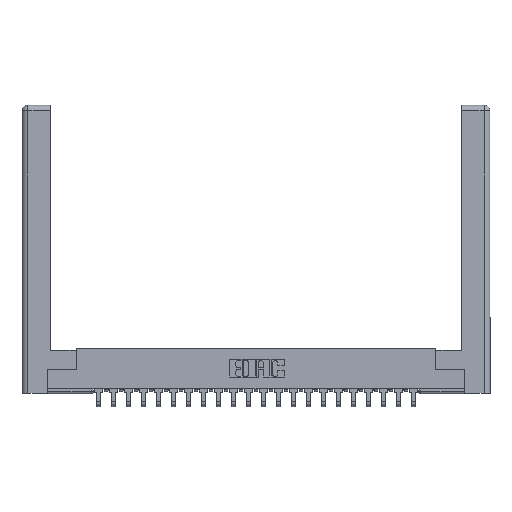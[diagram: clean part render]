
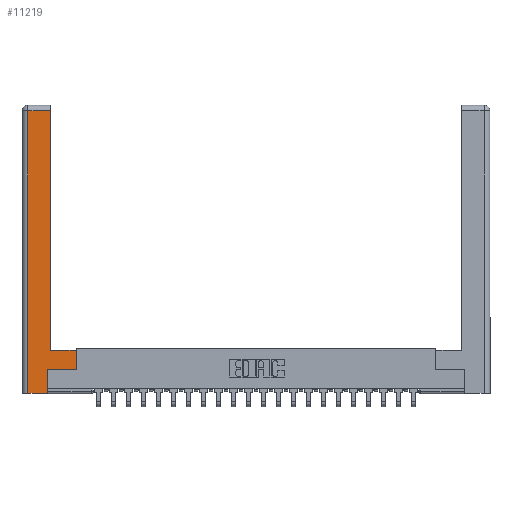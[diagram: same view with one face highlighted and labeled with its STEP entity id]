
A CAD part, top view. The second image highlights one B-rep face of the part: STEP entity #11219.
In plain terms, the highlighted planar face has unit normal (0, 0, 1).
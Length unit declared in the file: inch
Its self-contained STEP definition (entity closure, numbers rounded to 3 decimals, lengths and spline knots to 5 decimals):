
#249 = CARTESIAN_POINT ( 'NONE',  ( 0.265, 0.245, 0. ) ) ;
#416 = VECTOR ( 'NONE', #13026, 39.37008 ) ;
#850 = DIRECTION ( 'NONE',  ( 0., 1., 0. ) ) ;
#960 = VECTOR ( 'NONE', #8454, 39.37008 ) ;
#1880 = ORIENTED_EDGE ( 'NONE', *, *, #22420, .T. ) ;
#1926 = CARTESIAN_POINT ( 'NONE',  ( 0.295, 2.94, 0. ) ) ;
#2036 = LINE ( 'NONE', #17724, #17141 ) ;
#2659 = ORIENTED_EDGE ( 'NONE', *, *, #13560, .T. ) ;
#2972 = DIRECTION ( 'NONE',  ( 1., 0., 0. ) ) ;
#3571 = EDGE_CURVE ( 'NONE', #18539, #9554, #7698, .T. ) ;
#4336 = DIRECTION ( 'NONE',  ( 1., 0., 0. ) ) ;
#4462 = VERTEX_POINT ( 'NONE', #1926 ) ;
#5749 = ORIENTED_EDGE ( 'NONE', *, *, #9515, .T. ) ;
#5906 = LINE ( 'NONE', #19594, #960 ) ;
#6260 = EDGE_CURVE ( 'NONE', #16637, #12962, #2036, .T. ) ;
#6638 = CARTESIAN_POINT ( 'NONE',  ( 0.0615, 0., 0. ) ) ;
#6993 = LINE ( 'NONE', #19437, #16302 ) ;
#7064 = ORIENTED_EDGE ( 'NONE', *, *, #6260, .T. ) ;
#7620 = VECTOR ( 'NONE', #4336, 39.37008 ) ;
#7698 = LINE ( 'NONE', #11006, #416 ) ;
#7737 = CARTESIAN_POINT ( 'NONE',  ( 0.0615, 0., 0. ) ) ;
#8075 = LINE ( 'NONE', #16830, #17654 ) ;
#8365 = VERTEX_POINT ( 'NONE', #20976 ) ;
#8407 = ORIENTED_EDGE ( 'NONE', *, *, #18143, .T. ) ;
#8454 = DIRECTION ( 'NONE',  ( -1., 0., 0. ) ) ;
#9093 = VECTOR ( 'NONE', #23671, 39.37008 ) ;
#9161 = VERTEX_POINT ( 'NONE', #6638 ) ;
#9281 = LINE ( 'NONE', #7737, #20624 ) ;
#9515 = EDGE_CURVE ( 'NONE', #19848, #9161, #9281, .T. ) ;
#9554 = VERTEX_POINT ( 'NONE', #11461 ) ;
#10662 = CARTESIAN_POINT ( 'NONE',  ( 0.295, 0.45, 0. ) ) ;
#11006 = CARTESIAN_POINT ( 'NONE',  ( 0.565, 0.45, 0. ) ) ;
#11216 = CARTESIAN_POINT ( 'NONE',  ( 0.265, 0., 0. ) ) ;
#11219 = ADVANCED_FACE ( 'NONE', ( #20068 ), #15937, .F. ) ;
#11461 = CARTESIAN_POINT ( 'NONE',  ( 0.565, 0.45, 0. ) ) ;
#12962 = VERTEX_POINT ( 'NONE', #249 ) ;
#13026 = DIRECTION ( 'NONE',  ( 0., 1., 0. ) ) ;
#13560 = EDGE_CURVE ( 'NONE', #8365, #4462, #8075, .T. ) ;
#15061 = DIRECTION ( 'NONE',  ( 0., -1., 0. ) ) ;
#15487 = CARTESIAN_POINT ( 'NONE',  ( 0.265, 0., 0. ) ) ;
#15937 = PLANE ( 'NONE',  #15967 ) ;
#15967 = AXIS2_PLACEMENT_3D ( 'NONE', #21532, #17688, #17778 ) ;
#16302 = VECTOR ( 'NONE', #2972, 39.37008 ) ;
#16522 = EDGE_CURVE ( 'NONE', #9554, #8365, #18076, .T. ) ;
#16637 = VERTEX_POINT ( 'NONE', #11216 ) ;
#16830 = CARTESIAN_POINT ( 'NONE',  ( 0.295, 3., 0. ) ) ;
#16911 = CARTESIAN_POINT ( 'NONE',  ( 0.565, 0.245, 0. ) ) ;
#17141 = VECTOR ( 'NONE', #850, 39.37008 ) ;
#17654 = VECTOR ( 'NONE', #18765, 39.37008 ) ;
#17688 = DIRECTION ( 'NONE',  ( 0., 0., -1. ) ) ;
#17724 = CARTESIAN_POINT ( 'NONE',  ( 0.265, 0.245, 0. ) ) ;
#17778 = DIRECTION ( 'NONE',  ( -1., 0., 0. ) ) ;
#18076 = LINE ( 'NONE', #10662, #9093 ) ;
#18143 = EDGE_CURVE ( 'NONE', #12962, #18539, #6993, .T. ) ;
#18539 = VERTEX_POINT ( 'NONE', #16911 ) ;
#18765 = DIRECTION ( 'NONE',  ( 0., 1., 0. ) ) ;
#19437 = CARTESIAN_POINT ( 'NONE',  ( 0.565, 0.245, 0. ) ) ;
#19594 = CARTESIAN_POINT ( 'NONE',  ( 0.0615, 2.94, 0. ) ) ;
#19848 = VERTEX_POINT ( 'NONE', #20509 ) ;
#20068 = FACE_OUTER_BOUND ( 'NONE', #20530, .T. ) ;
#20509 = CARTESIAN_POINT ( 'NONE',  ( 0.0615, 2.94, 0. ) ) ;
#20530 = EDGE_LOOP ( 'NONE', ( #2659, #1880, #5749, #21576, #7064, #8407, #23846, #21151 ) ) ;
#20624 = VECTOR ( 'NONE', #15061, 39.37008 ) ;
#20970 = LINE ( 'NONE', #15487, #7620 ) ;
#20976 = CARTESIAN_POINT ( 'NONE',  ( 0.295, 0.45, 0. ) ) ;
#21151 = ORIENTED_EDGE ( 'NONE', *, *, #16522, .T. ) ;
#21532 = CARTESIAN_POINT ( 'NONE',  ( 0., 0., 0. ) ) ;
#21576 = ORIENTED_EDGE ( 'NONE', *, *, #23995, .T. ) ;
#22420 = EDGE_CURVE ( 'NONE', #4462, #19848, #5906, .T. ) ;
#23671 = DIRECTION ( 'NONE',  ( -1., 0., 0. ) ) ;
#23846 = ORIENTED_EDGE ( 'NONE', *, *, #3571, .T. ) ;
#23995 = EDGE_CURVE ( 'NONE', #9161, #16637, #20970, .T. ) ;
